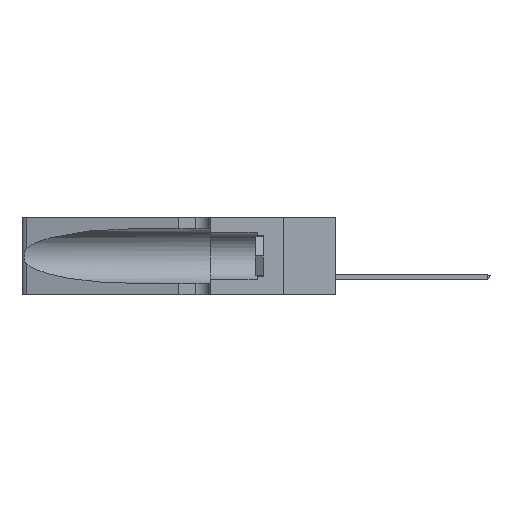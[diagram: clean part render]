
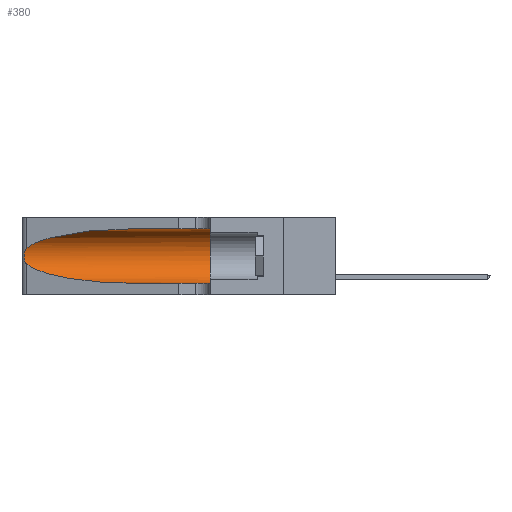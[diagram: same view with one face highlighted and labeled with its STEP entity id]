
A CAD part, left-side view. The second image highlights one B-rep face of the part: STEP entity #380.
In plain terms, the highlighted cylindrical face has radius 3.308 mm (diameter 6.617 mm), a partial arc.
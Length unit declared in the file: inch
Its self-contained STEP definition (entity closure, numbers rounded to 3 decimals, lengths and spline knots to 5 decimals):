
#162 = VERTEX_POINT ( 'NONE', #26112 ) ;
#380 = ADVANCED_FACE ( 'NONE', ( #39405 ), #26851, .F. ) ;
#411 = AXIS2_PLACEMENT_3D ( 'NONE', #16447, #7626, #19405 ) ;
#1078 = CARTESIAN_POINT ( 'NONE',  ( 0.2373, 1.15595, 0.08982 ) ) ;
#1943 = B_SPLINE_CURVE_WITH_KNOTS ( 'NONE', 3,
 ( #7506, #10429, #10302, #25959, #3987, #28911, #19424, #28645, #28778, #22525, #25701, #16847, #31757, #37948 ),
 .UNSPECIFIED., .F., .F.,
 ( 4, 2, 2, 2, 2, 2, 4 ),
 ( 0., 0.00027, 0.00053, 0.00107, 0.0016, 0.00187, 0.00214 ),
 .UNSPECIFIED. ) ;
#2380 = LINE ( 'NONE', #9521, #37941 ) ;
#3987 = CARTESIAN_POINT ( 'NONE',  ( 0.25854, 1.2359, 0.20912 ) ) ;
#4109 = CARTESIAN_POINT ( 'NONE',  ( 0.18966, 0.96281, 0.31525 ) ) ;
#4160 = CARTESIAN_POINT ( 'NONE',  ( 0.1305, 0.72297, 0.05475 ) ) ;
#5329 = EDGE_CURVE ( 'NONE', #162, #12367, #6349, .T. ) ;
#6126 = CIRCLE ( 'NONE', #411, 0.13025 ) ;
#6349 = LINE ( 'NONE', #31617, #23158 ) ;
#6946 = EDGE_CURVE ( 'NONE', #9191, #19120, #1943, .T. ) ;
#7506 = CARTESIAN_POINT ( 'NONE',  ( 0.25487, 1.22718, 0.22369 ) ) ;
#7626 = DIRECTION ( 'NONE',  ( 0., 1., 0. ) ) ;
#8923 = EDGE_CURVE ( 'NONE', #162, #9191, #19931, .T. ) ;
#9191 = VERTEX_POINT ( 'NONE', #36240 ) ;
#9521 = CARTESIAN_POINT ( 'NONE',  ( 0.1305, 1.61858, 0.05475 ) ) ;
#10302 = CARTESIAN_POINT ( 'NONE',  ( 0.25639, 1.23184, 0.21858 ) ) ;
#10429 = CARTESIAN_POINT ( 'NONE',  ( 0.25555, 1.22994, 0.2215 ) ) ;
#12367 = VERTEX_POINT ( 'NONE', #22256 ) ;
#12417 = ORIENTED_EDGE ( 'NONE', *, *, #37420, .F. ) ;
#13267 =( BOUNDED_CURVE ( )  B_SPLINE_CURVE ( 3, ( #22815, #1078, #22562, #4160 ),
 .UNSPECIFIED., .F., .T. ) 
 B_SPLINE_CURVE_WITH_KNOTS ( ( 4, 4 ),
 ( 3.44316, 4.71239 ),
 .UNSPECIFIED. ) 
 CURVE ( )  GEOMETRIC_REPRESENTATION_ITEM ( )  RATIONAL_B_SPLINE_CURVE ( ( 1., 0.87, 0.87, 1. ) ) 
 REPRESENTATION_ITEM ( '' )  );
#16126 = DIRECTION ( 'NONE',  ( 0., 0., -1. ) ) ;
#16447 = CARTESIAN_POINT ( 'NONE',  ( 0.1305, 0.35, 0.185 ) ) ;
#16586 = CARTESIAN_POINT ( 'NONE',  ( 0.1305, 0.72297, 0.31525 ) ) ;
#16847 = CARTESIAN_POINT ( 'NONE',  ( 0.25639, 1.23186, 0.15144 ) ) ;
#17992 = ORIENTED_EDGE ( 'NONE', *, *, #5329, .F. ) ;
#19120 = VERTEX_POINT ( 'NONE', #36297 ) ;
#19405 = DIRECTION ( 'NONE',  ( 0., 0., 1. ) ) ;
#19424 = CARTESIAN_POINT ( 'NONE',  ( 0.26075, 1.23896, 0.19203 ) ) ;
#19931 =( BOUNDED_CURVE ( )  B_SPLINE_CURVE ( 3, ( #16586, #4109, #25420, #38069 ),
 .UNSPECIFIED., .F., .T. ) 
 B_SPLINE_CURVE_WITH_KNOTS ( ( 4, 4 ),
 ( 1.5708, 2.84003 ),
 .UNSPECIFIED. ) 
 CURVE ( )  GEOMETRIC_REPRESENTATION_ITEM ( )  RATIONAL_B_SPLINE_CURVE ( ( 1., 0.87, 0.87, 1. ) ) 
 REPRESENTATION_ITEM ( '' )  );
#20010 = EDGE_CURVE ( 'NONE', #19120, #20461, #13267, .T. ) ;
#20382 = VERTEX_POINT ( 'NONE', #24373 ) ;
#20461 = VERTEX_POINT ( 'NONE', #37023 ) ;
#20789 = EDGE_LOOP ( 'NONE', ( #31620, #38016, #26569, #37635, #12417, #17992 ) ) ;
#21163 = DIRECTION ( 'NONE',  ( 0., -1., 0. ) ) ;
#22256 = CARTESIAN_POINT ( 'NONE',  ( 0.1305, 0.35, 0.31525 ) ) ;
#22270 = DIRECTION ( 'NONE',  ( 0., -1., 0. ) ) ;
#22453 = CARTESIAN_POINT ( 'NONE',  ( 0.1305, 1.61858, 0.185 ) ) ;
#22525 = CARTESIAN_POINT ( 'NONE',  ( 0.25856, 1.23593, 0.16098 ) ) ;
#22562 = CARTESIAN_POINT ( 'NONE',  ( 0.18966, 0.96281, 0.05475 ) ) ;
#22815 = CARTESIAN_POINT ( 'NONE',  ( 0.25487, 1.22718, 0.14631 ) ) ;
#23158 = VECTOR ( 'NONE', #21163, 39.37008 ) ;
#24373 = CARTESIAN_POINT ( 'NONE',  ( 0.1305, 0.35, 0.05475 ) ) ;
#25420 = CARTESIAN_POINT ( 'NONE',  ( 0.2373, 1.15595, 0.28018 ) ) ;
#25701 = CARTESIAN_POINT ( 'NONE',  ( 0.25789, 1.23486, 0.15765 ) ) ;
#25959 = CARTESIAN_POINT ( 'NONE',  ( 0.25787, 1.23484, 0.2124 ) ) ;
#26112 = CARTESIAN_POINT ( 'NONE',  ( 0.1305, 0.72297, 0.31525 ) ) ;
#26569 = ORIENTED_EDGE ( 'NONE', *, *, #20010, .T. ) ;
#26851 = CYLINDRICAL_SURFACE ( 'NONE', #38612, 0.13025 ) ;
#28645 = CARTESIAN_POINT ( 'NONE',  ( 0.26075, 1.23896, 0.178 ) ) ;
#28778 = CARTESIAN_POINT ( 'NONE',  ( 0.26017, 1.23833, 0.17102 ) ) ;
#28911 = CARTESIAN_POINT ( 'NONE',  ( 0.26018, 1.23835, 0.19895 ) ) ;
#31617 = CARTESIAN_POINT ( 'NONE',  ( 0.1305, 1.61858, 0.31525 ) ) ;
#31620 = ORIENTED_EDGE ( 'NONE', *, *, #8923, .T. ) ;
#31757 = CARTESIAN_POINT ( 'NONE',  ( 0.25555, 1.22993, 0.14849 ) ) ;
#32934 = EDGE_CURVE ( 'NONE', #20461, #20382, #2380, .T. ) ;
#36240 = CARTESIAN_POINT ( 'NONE',  ( 0.25487, 1.22718, 0.22369 ) ) ;
#36297 = CARTESIAN_POINT ( 'NONE',  ( 0.25487, 1.22718, 0.14631 ) ) ;
#37023 = CARTESIAN_POINT ( 'NONE',  ( 0.1305, 0.72297, 0.05475 ) ) ;
#37420 = EDGE_CURVE ( 'NONE', #12367, #20382, #6126, .T. ) ;
#37635 = ORIENTED_EDGE ( 'NONE', *, *, #32934, .T. ) ;
#37880 = DIRECTION ( 'NONE',  ( 0., -1., 0. ) ) ;
#37941 = VECTOR ( 'NONE', #22270, 39.37008 ) ;
#37948 = CARTESIAN_POINT ( 'NONE',  ( 0.25487, 1.22718, 0.14631 ) ) ;
#38016 = ORIENTED_EDGE ( 'NONE', *, *, #6946, .T. ) ;
#38069 = CARTESIAN_POINT ( 'NONE',  ( 0.25487, 1.22718, 0.22369 ) ) ;
#38612 = AXIS2_PLACEMENT_3D ( 'NONE', #22453, #37880, #16126 ) ;
#39405 = FACE_OUTER_BOUND ( 'NONE', #20789, .T. ) ;
